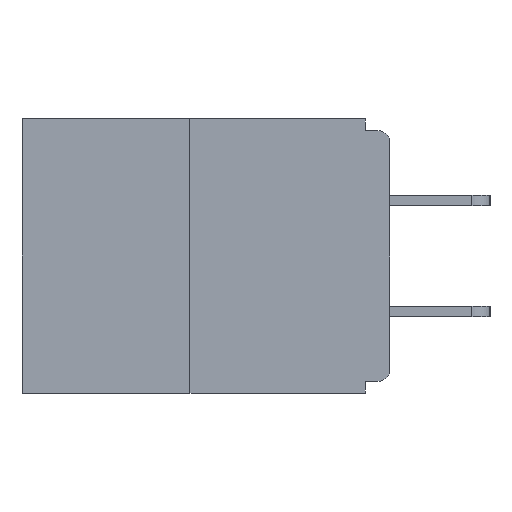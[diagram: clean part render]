
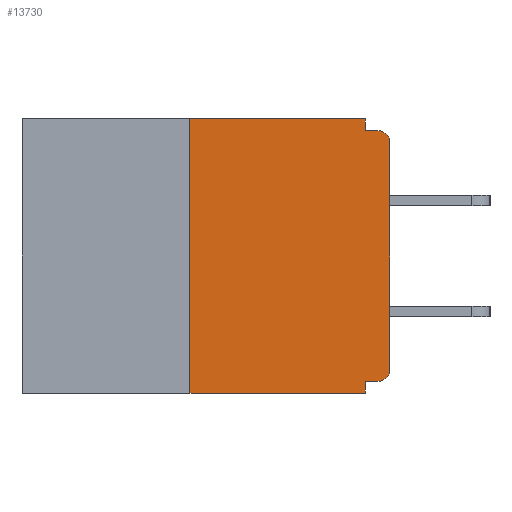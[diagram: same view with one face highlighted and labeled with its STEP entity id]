
A CAD part, left-side view. The second image highlights one B-rep face of the part: STEP entity #13730.
In plain terms, the highlighted planar face has unit normal (-1, 0, 0).
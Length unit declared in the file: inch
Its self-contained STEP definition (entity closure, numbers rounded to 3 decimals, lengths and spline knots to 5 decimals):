
#145 = ORIENTED_EDGE ( 'NONE', *, *, #14674, .F. ) ;
#433 = VECTOR ( 'NONE', #20304, 39.37008 ) ;
#576 = ORIENTED_EDGE ( 'NONE', *, *, #19466, .T. ) ;
#1561 = CARTESIAN_POINT ( 'NONE',  ( 0., 0.015, -0.015 ) ) ;
#1797 = CARTESIAN_POINT ( 'NONE',  ( 0., 0.031, 0. ) ) ;
#2094 = EDGE_CURVE ( 'NONE', #16967, #21814, #11352, .T. ) ;
#2323 = CARTESIAN_POINT ( 'NONE',  ( 0., 0.031, -0.015 ) ) ;
#2646 = EDGE_CURVE ( 'NONE', #28146, #3461, #22770, .T. ) ;
#2681 = DIRECTION ( 'NONE',  ( 0., 1., 0. ) ) ;
#2729 = CARTESIAN_POINT ( 'NONE',  ( 0., 0.46, 0. ) ) ;
#3386 = LINE ( 'NONE', #25887, #25307 ) ;
#3461 = VERTEX_POINT ( 'NONE', #1561 ) ;
#3623 = EDGE_CURVE ( 'NONE', #9005, #21814, #15253, .T. ) ;
#4337 = EDGE_LOOP ( 'NONE', ( #145, #27393, #24319, #12254, #13614, #576, #5141, #21170, #6511, #18041 ) ) ;
#5141 = ORIENTED_EDGE ( 'NONE', *, *, #5621, .T. ) ;
#5621 = EDGE_CURVE ( 'NONE', #18418, #28146, #3386, .T. ) ;
#5635 = CARTESIAN_POINT ( 'NONE',  ( 0., 0.015, -0.313 ) ) ;
#6296 = FACE_OUTER_BOUND ( 'NONE', #4337, .T. ) ;
#6511 = ORIENTED_EDGE ( 'NONE', *, *, #20881, .F. ) ;
#7288 = LINE ( 'NONE', #11612, #9588 ) ;
#7571 = DIRECTION ( 'NONE',  ( -1., 0., 0. ) ) ;
#8049 = EDGE_CURVE ( 'NONE', #22090, #16967, #7288, .T. ) ;
#8634 = AXIS2_PLACEMENT_3D ( 'NONE', #17673, #17807, #26607 ) ;
#8732 = VECTOR ( 'NONE', #20795, 39.37008 ) ;
#8752 = CARTESIAN_POINT ( 'NONE',  ( 0., 0.46, -0.343 ) ) ;
#9005 = VERTEX_POINT ( 'NONE', #14286 ) ;
#9588 = VECTOR ( 'NONE', #2681, 39.37008 ) ;
#10580 = LINE ( 'NONE', #1797, #25362 ) ;
#11039 = PLANE ( 'NONE',  #8634 ) ;
#11352 = LINE ( 'NONE', #20157, #433 ) ;
#11612 = CARTESIAN_POINT ( 'NONE',  ( 0., 0., -0.328 ) ) ;
#11718 = AXIS2_PLACEMENT_3D ( 'NONE', #27319, #7571, #16367 ) ;
#12254 = ORIENTED_EDGE ( 'NONE', *, *, #2094, .F. ) ;
#12325 = CARTESIAN_POINT ( 'NONE',  ( 0., 0.25, 0. ) ) ;
#12972 = CARTESIAN_POINT ( 'NONE',  ( 0., 0., -0.03 ) ) ;
#13614 = ORIENTED_EDGE ( 'NONE', *, *, #8049, .F. ) ;
#13730 = ADVANCED_FACE ( 'NONE', ( #6296 ), #11039, .F. ) ;
#14286 = CARTESIAN_POINT ( 'NONE',  ( 0., 0.25, -0.343 ) ) ;
#14446 = LINE ( 'NONE', #22942, #8732 ) ;
#14674 = EDGE_CURVE ( 'NONE', #27317, #19251, #22620, .T. ) ;
#14934 = DIRECTION ( 'NONE',  ( 0., 0., 1. ) ) ;
#15055 = DIRECTION ( 'NONE',  ( 0., 0., 1. ) ) ;
#15253 = LINE ( 'NONE', #8752, #17067 ) ;
#16367 = DIRECTION ( 'NONE',  ( 0., 0., -1. ) ) ;
#16617 = CARTESIAN_POINT ( 'NONE',  ( 0., 0.015, -0.328 ) ) ;
#16967 = VERTEX_POINT ( 'NONE', #25587 ) ;
#17067 = VECTOR ( 'NONE', #19861, 39.37008 ) ;
#17080 = LINE ( 'NONE', #17215, #23983 ) ;
#17215 = CARTESIAN_POINT ( 'NONE',  ( 0., 0.25, 0. ) ) ;
#17673 = CARTESIAN_POINT ( 'NONE',  ( 0., 0.46, 0. ) ) ;
#17807 = DIRECTION ( 'NONE',  ( 1., 0., 0. ) ) ;
#17852 = VERTEX_POINT ( 'NONE', #2323 ) ;
#18041 = ORIENTED_EDGE ( 'NONE', *, *, #21759, .F. ) ;
#18418 = VERTEX_POINT ( 'NONE', #19877 ) ;
#19251 = VERTEX_POINT ( 'NONE', #23693 ) ;
#19466 = EDGE_CURVE ( 'NONE', #22090, #18418, #20718, .T. ) ;
#19663 = DIRECTION ( 'NONE',  ( 0., 0., -1. ) ) ;
#19861 = DIRECTION ( 'NONE',  ( 0., -1., 0. ) ) ;
#19877 = CARTESIAN_POINT ( 'NONE',  ( 0., 0., -0.313 ) ) ;
#20157 = CARTESIAN_POINT ( 'NONE',  ( 0., 0.031, -0.343 ) ) ;
#20304 = DIRECTION ( 'NONE',  ( 0., 0., -1. ) ) ;
#20323 = DIRECTION ( 'NONE',  ( 0., -1., 0. ) ) ;
#20718 = CIRCLE ( 'NONE', #25251, 0.015 ) ;
#20795 = DIRECTION ( 'NONE',  ( 0., -1., 0. ) ) ;
#20881 = EDGE_CURVE ( 'NONE', #17852, #3461, #14446, .T. ) ;
#21170 = ORIENTED_EDGE ( 'NONE', *, *, #2646, .T. ) ;
#21759 = EDGE_CURVE ( 'NONE', #19251, #17852, #10580, .T. ) ;
#21814 = VERTEX_POINT ( 'NONE', #24262 ) ;
#21816 = EDGE_CURVE ( 'NONE', #9005, #27317, #17080, .T. ) ;
#22090 = VERTEX_POINT ( 'NONE', #16617 ) ;
#22620 = LINE ( 'NONE', #2729, #28031 ) ;
#22770 = CIRCLE ( 'NONE', #11718, 0.015 ) ;
#22795 = DIRECTION ( 'NONE',  ( -1., 0., 0. ) ) ;
#22942 = CARTESIAN_POINT ( 'NONE',  ( 0., 0., -0.015 ) ) ;
#23693 = CARTESIAN_POINT ( 'NONE',  ( 0., 0.031, 0. ) ) ;
#23983 = VECTOR ( 'NONE', #15055, 39.37008 ) ;
#24262 = CARTESIAN_POINT ( 'NONE',  ( 0., 0.031, -0.343 ) ) ;
#24319 = ORIENTED_EDGE ( 'NONE', *, *, #3623, .T. ) ;
#25099 = DIRECTION ( 'NONE',  ( 0., 0., -1. ) ) ;
#25251 = AXIS2_PLACEMENT_3D ( 'NONE', #5635, #22795, #25099 ) ;
#25307 = VECTOR ( 'NONE', #14934, 39.37008 ) ;
#25362 = VECTOR ( 'NONE', #19663, 39.37008 ) ;
#25587 = CARTESIAN_POINT ( 'NONE',  ( 0., 0.031, -0.328 ) ) ;
#25887 = CARTESIAN_POINT ( 'NONE',  ( 0., 0., 0. ) ) ;
#26607 = DIRECTION ( 'NONE',  ( 0., 0., -1. ) ) ;
#27317 = VERTEX_POINT ( 'NONE', #12325 ) ;
#27319 = CARTESIAN_POINT ( 'NONE',  ( 0., 0.015, -0.03 ) ) ;
#27393 = ORIENTED_EDGE ( 'NONE', *, *, #21816, .F. ) ;
#28031 = VECTOR ( 'NONE', #20323, 39.37008 ) ;
#28146 = VERTEX_POINT ( 'NONE', #12972 ) ;
